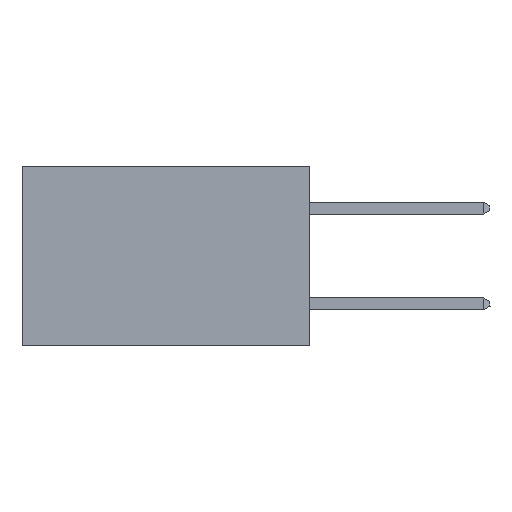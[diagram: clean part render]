
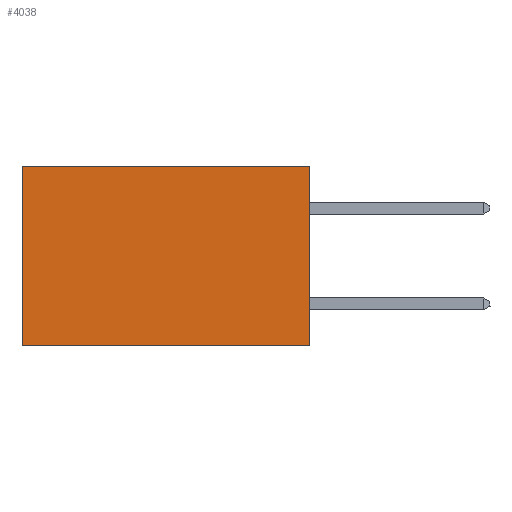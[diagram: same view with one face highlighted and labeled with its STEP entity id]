
A CAD part, left-side view. The second image highlights one B-rep face of the part: STEP entity #4038.
In plain terms, the highlighted planar face has unit normal (-1, 0, 0).
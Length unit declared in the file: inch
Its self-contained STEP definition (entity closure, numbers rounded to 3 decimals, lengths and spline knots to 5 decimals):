
#530 = DIRECTION ( 'NONE',  ( 0., 0., -1. ) ) ;
#548 = ORIENTED_EDGE ( 'NONE', *, *, #15020, .T. ) ;
#554 = LINE ( 'NONE', #6059, #1824 ) ;
#861 = LINE ( 'NONE', #1803, #10918 ) ;
#997 = EDGE_CURVE ( 'NONE', #8436, #15455, #861, .T. ) ;
#1016 = CARTESIAN_POINT ( 'NONE',  ( 0.2875, 0.6, 0. ) ) ;
#1458 = PLANE ( 'NONE',  #13997 ) ;
#1803 = CARTESIAN_POINT ( 'NONE',  ( 0.2875, 0., -0.375 ) ) ;
#1824 = VECTOR ( 'NONE', #2652, 39.37008 ) ;
#2025 = VERTEX_POINT ( 'NONE', #6801 ) ;
#2652 = DIRECTION ( 'NONE',  ( 0., 0., -1. ) ) ;
#2998 = EDGE_LOOP ( 'NONE', ( #12709, #9734, #12720, #548 ) ) ;
#3403 = CARTESIAN_POINT ( 'NONE',  ( 0.2875, 0., -0.375 ) ) ;
#3582 = EDGE_CURVE ( 'NONE', #2025, #8436, #554, .T. ) ;
#3955 = CARTESIAN_POINT ( 'NONE',  ( 0.2875, 0.6, -0.375 ) ) ;
#4038 = ADVANCED_FACE ( 'NONE', ( #6266 ), #1458, .F. ) ;
#4529 = DIRECTION ( 'NONE',  ( 0., 1., 0. ) ) ;
#4798 = LINE ( 'NONE', #14195, #7579 ) ;
#6059 = CARTESIAN_POINT ( 'NONE',  ( 0.2875, 0., -0.375 ) ) ;
#6174 = DIRECTION ( 'NONE',  ( 0., 0., -1. ) ) ;
#6266 = FACE_OUTER_BOUND ( 'NONE', #2998, .T. ) ;
#6801 = CARTESIAN_POINT ( 'NONE',  ( 0.2875, 0., 0. ) ) ;
#6989 = VERTEX_POINT ( 'NONE', #1016 ) ;
#7579 = VECTOR ( 'NONE', #4529, 39.37008 ) ;
#8436 = VERTEX_POINT ( 'NONE', #3403 ) ;
#8511 = CARTESIAN_POINT ( 'NONE',  ( 0.2875, 0.6, -0.375 ) ) ;
#9031 = DIRECTION ( 'NONE',  ( 0., 1., 0. ) ) ;
#9310 = VECTOR ( 'NONE', #530, 39.37008 ) ;
#9734 = ORIENTED_EDGE ( 'NONE', *, *, #997, .F. ) ;
#9837 = CARTESIAN_POINT ( 'NONE',  ( 0.2875, 0., -0.375 ) ) ;
#10918 = VECTOR ( 'NONE', #9031, 39.37008 ) ;
#12460 = LINE ( 'NONE', #3955, #9310 ) ;
#12709 = ORIENTED_EDGE ( 'NONE', *, *, #15110, .T. ) ;
#12720 = ORIENTED_EDGE ( 'NONE', *, *, #3582, .F. ) ;
#13997 = AXIS2_PLACEMENT_3D ( 'NONE', #9837, #14524, #6174 ) ;
#14195 = CARTESIAN_POINT ( 'NONE',  ( 0.2875, 0., 0. ) ) ;
#14524 = DIRECTION ( 'NONE',  ( 1., 0., 0. ) ) ;
#15020 = EDGE_CURVE ( 'NONE', #2025, #6989, #4798, .T. ) ;
#15110 = EDGE_CURVE ( 'NONE', #6989, #15455, #12460, .T. ) ;
#15455 = VERTEX_POINT ( 'NONE', #8511 ) ;
